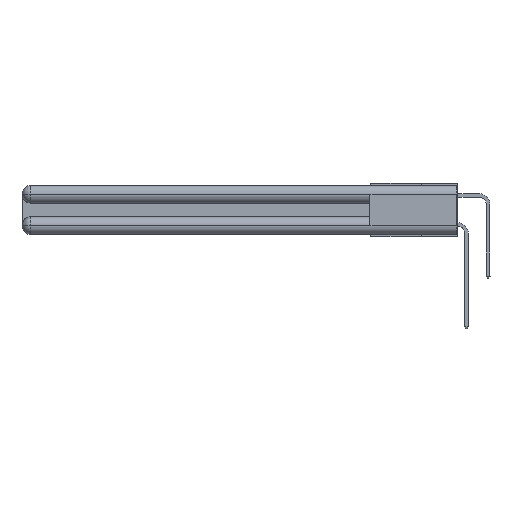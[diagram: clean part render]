
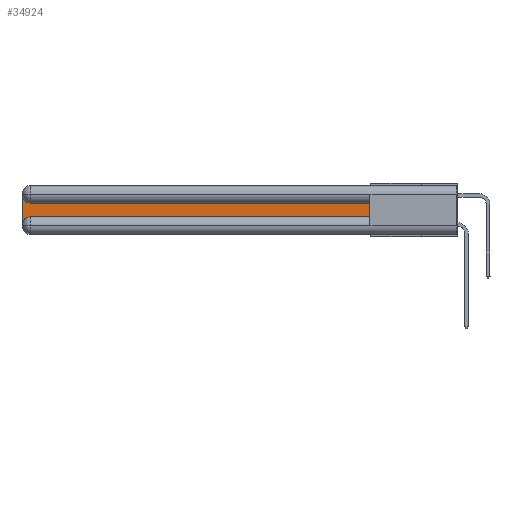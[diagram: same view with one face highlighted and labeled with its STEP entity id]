
A CAD part, left-side view. The second image highlights one B-rep face of the part: STEP entity #34924.
In plain terms, the highlighted planar face has unit normal (-1, 0, 0).
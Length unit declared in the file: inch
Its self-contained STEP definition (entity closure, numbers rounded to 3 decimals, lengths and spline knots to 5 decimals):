
#1950 = CARTESIAN_POINT ( 'NONE',  ( 0.075, 0.6, -0.2175 ) ) ;
#2211 = AXIS2_PLACEMENT_3D ( 'NONE', #34890, #18028, #26506 ) ;
#3186 = ORIENTED_EDGE ( 'NONE', *, *, #23118, .T. ) ;
#3408 = VECTOR ( 'NONE', #29127, 39.37008 ) ;
#3874 = DIRECTION ( 'NONE',  ( 0., 0., -1. ) ) ;
#4168 = CARTESIAN_POINT ( 'NONE',  ( 0.075, 0.6, -0.1225 ) ) ;
#4820 = VERTEX_POINT ( 'NONE', #24256 ) ;
#5563 = LINE ( 'NONE', #1950, #7262 ) ;
#5818 = FACE_OUTER_BOUND ( 'NONE', #15444, .T. ) ;
#5847 = CIRCLE ( 'NONE', #33163, 0.06 ) ;
#7262 = VECTOR ( 'NONE', #18384, 39.37008 ) ;
#7689 = LINE ( 'NONE', #23400, #8598 ) ;
#8258 = CARTESIAN_POINT ( 'NONE',  ( 0.075, 3., -0.2775 ) ) ;
#8598 = VECTOR ( 'NONE', #3874, 39.37008 ) ;
#8889 = ORIENTED_EDGE ( 'NONE', *, *, #18589, .T. ) ;
#8957 = DIRECTION ( 'NONE',  ( 1., 0., 0. ) ) ;
#9073 = ORIENTED_EDGE ( 'NONE', *, *, #19804, .T. ) ;
#9492 = DIRECTION ( 'NONE',  ( 0., 0., -1. ) ) ;
#10318 = AXIS2_PLACEMENT_3D ( 'NONE', #26302, #31920, #9492 ) ;
#10887 = LINE ( 'NONE', #17702, #3408 ) ;
#12298 = EDGE_CURVE ( 'NONE', #4820, #35746, #7689, .T. ) ;
#14187 = VERTEX_POINT ( 'NONE', #27935 ) ;
#15444 = EDGE_LOOP ( 'NONE', ( #3186, #9073, #23834, #21118, #22422, #8889 ) ) ;
#15630 = EDGE_CURVE ( 'NONE', #15746, #14187, #5563, .T. ) ;
#15746 = VERTEX_POINT ( 'NONE', #28226 ) ;
#16509 = LINE ( 'NONE', #4168, #29687 ) ;
#17702 = CARTESIAN_POINT ( 'NONE',  ( 0.075, 0.6, -0.2175 ) ) ;
#18028 = DIRECTION ( 'NONE',  ( 1., 0., 0. ) ) ;
#18047 = DIRECTION ( 'NONE',  ( 0., 1., 0. ) ) ;
#18384 = DIRECTION ( 'NONE',  ( 0., -1., 0. ) ) ;
#18589 = EDGE_CURVE ( 'NONE', #14187, #34811, #10887, .T. ) ;
#19804 = EDGE_CURVE ( 'NONE', #32089, #4820, #34152, .T. ) ;
#21118 = ORIENTED_EDGE ( 'NONE', *, *, #28089, .T. ) ;
#22422 = ORIENTED_EDGE ( 'NONE', *, *, #15630, .T. ) ;
#23078 = CARTESIAN_POINT ( 'NONE',  ( 0.075, 2.94, -0.2775 ) ) ;
#23118 = EDGE_CURVE ( 'NONE', #34811, #32089, #16509, .T. ) ;
#23400 = CARTESIAN_POINT ( 'NONE',  ( 0.075, 3., -0.2175 ) ) ;
#23543 = DIRECTION ( 'NONE',  ( 0., 0., -1. ) ) ;
#23834 = ORIENTED_EDGE ( 'NONE', *, *, #12298, .T. ) ;
#24256 = CARTESIAN_POINT ( 'NONE',  ( 0.075, 3., -0.0625 ) ) ;
#25305 = CARTESIAN_POINT ( 'NONE',  ( 0.075, 2.94, -0.1225 ) ) ;
#26302 = CARTESIAN_POINT ( 'NONE',  ( 0.075, 3., -0.1225 ) ) ;
#26506 = DIRECTION ( 'NONE',  ( 0., 0., -1. ) ) ;
#27935 = CARTESIAN_POINT ( 'NONE',  ( 0.075, 0.6, -0.2175 ) ) ;
#28089 = EDGE_CURVE ( 'NONE', #35746, #15746, #5847, .T. ) ;
#28226 = CARTESIAN_POINT ( 'NONE',  ( 0.075, 2.94, -0.2175 ) ) ;
#29114 = PLANE ( 'NONE',  #10318 ) ;
#29127 = DIRECTION ( 'NONE',  ( 0., 0., 1. ) ) ;
#29687 = VECTOR ( 'NONE', #18047, 39.37008 ) ;
#31803 = CARTESIAN_POINT ( 'NONE',  ( 0.075, 0.6, -0.1225 ) ) ;
#31920 = DIRECTION ( 'NONE',  ( 1., 0., 0. ) ) ;
#32089 = VERTEX_POINT ( 'NONE', #25305 ) ;
#33163 = AXIS2_PLACEMENT_3D ( 'NONE', #23078, #8957, #23543 ) ;
#34152 = CIRCLE ( 'NONE', #2211, 0.06 ) ;
#34811 = VERTEX_POINT ( 'NONE', #31803 ) ;
#34890 = CARTESIAN_POINT ( 'NONE',  ( 0.075, 2.94, -0.0625 ) ) ;
#34924 = ADVANCED_FACE ( 'NONE', ( #5818 ), #29114, .F. ) ;
#35746 = VERTEX_POINT ( 'NONE', #8258 ) ;
